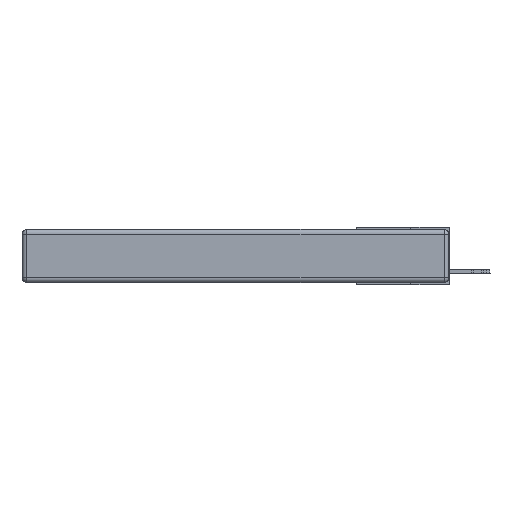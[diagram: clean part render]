
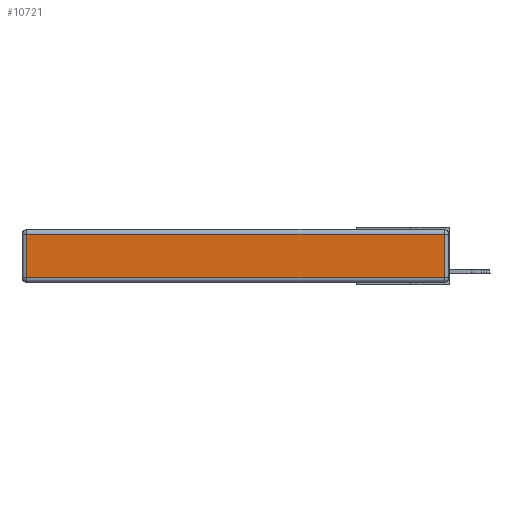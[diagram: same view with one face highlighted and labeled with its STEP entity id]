
A CAD part, left-side view. The second image highlights one B-rep face of the part: STEP entity #10721.
In plain terms, the highlighted planar face has unit normal (-1, 0, 0).
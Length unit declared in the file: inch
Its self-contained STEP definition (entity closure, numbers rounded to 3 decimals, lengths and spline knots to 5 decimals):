
#643 = DIRECTION ( 'NONE',  ( 0., 0., -1. ) ) ;
#941 = ORIENTED_EDGE ( 'NONE', *, *, #13802, .T. ) ;
#977 = CARTESIAN_POINT ( 'NONE',  ( 0., 0.03, -0.343 ) ) ;
#3148 = CARTESIAN_POINT ( 'NONE',  ( 0., 0., -0.313 ) ) ;
#3334 = DIRECTION ( 'NONE',  ( -1., 0., 0. ) ) ;
#3709 = DIRECTION ( 'NONE',  ( 0., 0., 1. ) ) ;
#4345 = LINE ( 'NONE', #12177, #12823 ) ;
#4365 = VECTOR ( 'NONE', #3709, 39.37008 ) ;
#5544 = FACE_OUTER_BOUND ( 'NONE', #13203, .T. ) ;
#8068 = CARTESIAN_POINT ( 'NONE',  ( 0., 0.03, -0.03 ) ) ;
#10194 = EDGE_CURVE ( 'NONE', #13504, #10656, #18071, .T. ) ;
#10656 = VERTEX_POINT ( 'NONE', #8068 ) ;
#10721 = ADVANCED_FACE ( 'NONE', ( #5544 ), #31222, .T. ) ;
#12177 = CARTESIAN_POINT ( 'NONE',  ( 0., 2.75, -0.03 ) ) ;
#12823 = VECTOR ( 'NONE', #17326, 39.37008 ) ;
#13203 = EDGE_LOOP ( 'NONE', ( #15784, #15648, #20741, #941 ) ) ;
#13504 = VERTEX_POINT ( 'NONE', #14171 ) ;
#13802 = EDGE_CURVE ( 'NONE', #17894, #14355, #16313, .T. ) ;
#14171 = CARTESIAN_POINT ( 'NONE',  ( 0., 0.03, -0.313 ) ) ;
#14355 = VERTEX_POINT ( 'NONE', #17955 ) ;
#15123 = VECTOR ( 'NONE', #643, 39.37008 ) ;
#15648 = ORIENTED_EDGE ( 'NONE', *, *, #10194, .T. ) ;
#15784 = ORIENTED_EDGE ( 'NONE', *, *, #24312, .T. ) ;
#16313 = LINE ( 'NONE', #31033, #15123 ) ;
#16415 = VECTOR ( 'NONE', #28883, 39.37008 ) ;
#17326 = DIRECTION ( 'NONE',  ( 0., 1., 0. ) ) ;
#17894 = VERTEX_POINT ( 'NONE', #26722 ) ;
#17955 = CARTESIAN_POINT ( 'NONE',  ( 0., 2.72, -0.313 ) ) ;
#18071 = LINE ( 'NONE', #977, #4365 ) ;
#18498 = EDGE_CURVE ( 'NONE', #10656, #17894, #4345, .T. ) ;
#18754 = DIRECTION ( 'NONE',  ( 0., 0., 1. ) ) ;
#20741 = ORIENTED_EDGE ( 'NONE', *, *, #18498, .T. ) ;
#23293 = LINE ( 'NONE', #3148, #16415 ) ;
#24229 = AXIS2_PLACEMENT_3D ( 'NONE', #25735, #3334, #18754 ) ;
#24312 = EDGE_CURVE ( 'NONE', #14355, #13504, #23293, .T. ) ;
#25735 = CARTESIAN_POINT ( 'NONE',  ( 0., 0., -0.343 ) ) ;
#26722 = CARTESIAN_POINT ( 'NONE',  ( 0., 2.72, -0.03 ) ) ;
#28883 = DIRECTION ( 'NONE',  ( 0., -1., 0. ) ) ;
#31033 = CARTESIAN_POINT ( 'NONE',  ( 0., 2.72, -0.343 ) ) ;
#31222 = PLANE ( 'NONE',  #24229 ) ;
